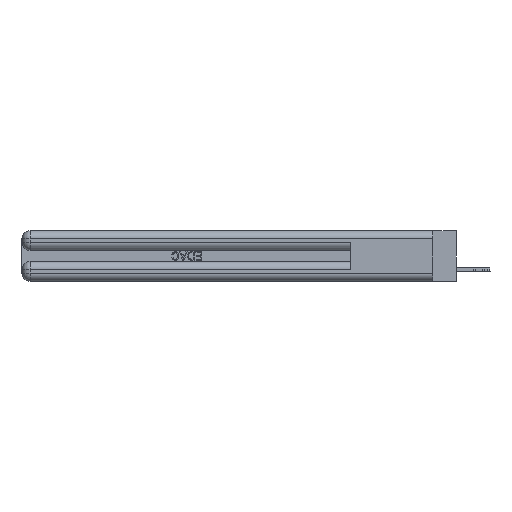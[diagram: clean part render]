
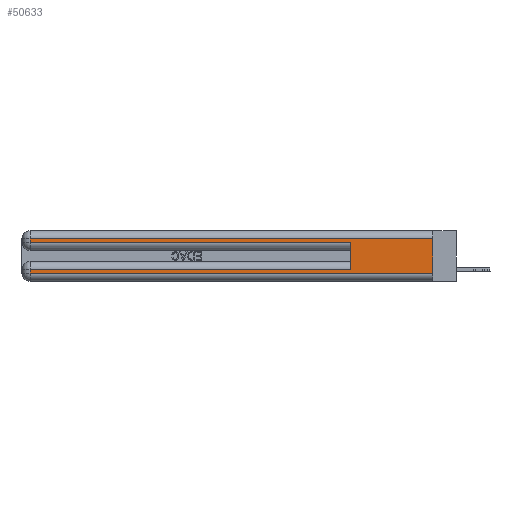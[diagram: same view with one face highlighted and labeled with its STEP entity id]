
A CAD part, left-side view. The second image highlights one B-rep face of the part: STEP entity #50633.
In plain terms, the highlighted planar face has unit normal (-1, 0, 0).
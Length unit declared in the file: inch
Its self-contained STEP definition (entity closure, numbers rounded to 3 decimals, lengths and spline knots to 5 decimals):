
#714 = VERTEX_POINT ( 'NONE', #5975 ) ;
#1698 = DIRECTION ( 'NONE',  ( 0., 0., -1. ) ) ;
#1939 = PLANE ( 'NONE',  #7676 ) ;
#3007 = EDGE_CURVE ( 'NONE', #8865, #45601, #22448, .T. ) ;
#3083 = CARTESIAN_POINT ( 'NONE',  ( 0., 0., 0.37 ) ) ;
#3136 = VECTOR ( 'NONE', #39559, 39.37008 ) ;
#4416 = LINE ( 'NONE', #47238, #3136 ) ;
#5319 = LINE ( 'NONE', #34522, #34477 ) ;
#5425 = VERTEX_POINT ( 'NONE', #7250 ) ;
#5836 = CARTESIAN_POINT ( 'NONE',  ( 0., 2.94, 0.37 ) ) ;
#5975 = CARTESIAN_POINT ( 'NONE',  ( 0., 2.94, 0.06 ) ) ;
#6812 = CARTESIAN_POINT ( 'NONE',  ( 0., 0., 0.31 ) ) ;
#7250 = CARTESIAN_POINT ( 'NONE',  ( 0., 2.94, 0.31 ) ) ;
#7676 = AXIS2_PLACEMENT_3D ( 'NONE', #3083, #44331, #23561 ) ;
#8230 = DIRECTION ( 'NONE',  ( 0., -1., 0. ) ) ;
#8388 = EDGE_CURVE ( 'NONE', #8865, #5425, #21188, .T. ) ;
#8865 = VERTEX_POINT ( 'NONE', #32283 ) ;
#9488 = DIRECTION ( 'NONE',  ( 0., 0., -1. ) ) ;
#10222 = LINE ( 'NONE', #5836, #36821 ) ;
#10442 = CARTESIAN_POINT ( 'NONE',  ( 0., 0., 0.285 ) ) ;
#12274 = DIRECTION ( 'NONE',  ( 0., 1., 0. ) ) ;
#14746 = LINE ( 'NONE', #10442, #50846 ) ;
#15194 = LINE ( 'NONE', #31770, #40395 ) ;
#18966 = CARTESIAN_POINT ( 'NONE',  ( 0., 0., 0.37 ) ) ;
#20331 = EDGE_LOOP ( 'NONE', ( #33616, #41863, #33061, #52438, #41992, #24091, #39143, #36077 ) ) ;
#20453 = VERTEX_POINT ( 'NONE', #47409 ) ;
#20526 = EDGE_CURVE ( 'NONE', #20453, #39081, #14746, .T. ) ;
#20654 = EDGE_CURVE ( 'NONE', #5425, #20453, #10222, .T. ) ;
#21188 = LINE ( 'NONE', #6812, #49023 ) ;
#22448 = LINE ( 'NONE', #18966, #41895 ) ;
#23075 = EDGE_CURVE ( 'NONE', #43983, #714, #5319, .T. ) ;
#23313 = DIRECTION ( 'NONE',  ( 0., 1., 0. ) ) ;
#23561 = DIRECTION ( 'NONE',  ( 0., 0., -1. ) ) ;
#23565 = CARTESIAN_POINT ( 'NONE',  ( 0., 2.94, 0.085 ) ) ;
#24091 = ORIENTED_EDGE ( 'NONE', *, *, #29529, .T. ) ;
#25973 = EDGE_CURVE ( 'NONE', #32829, #39081, #4416, .T. ) ;
#27393 = LINE ( 'NONE', #28270, #36499 ) ;
#28270 = CARTESIAN_POINT ( 'NONE',  ( 0., 0., 0.085 ) ) ;
#29035 = EDGE_CURVE ( 'NONE', #714, #45601, #15194, .T. ) ;
#29337 = CARTESIAN_POINT ( 'NONE',  ( 0., 0., 0.06 ) ) ;
#29529 = EDGE_CURVE ( 'NONE', #32829, #43983, #27393, .T. ) ;
#31770 = CARTESIAN_POINT ( 'NONE',  ( 0., 0., 0.06 ) ) ;
#32283 = CARTESIAN_POINT ( 'NONE',  ( 0., 0., 0.31 ) ) ;
#32829 = VERTEX_POINT ( 'NONE', #52883 ) ;
#33061 = ORIENTED_EDGE ( 'NONE', *, *, #20654, .T. ) ;
#33616 = ORIENTED_EDGE ( 'NONE', *, *, #3007, .F. ) ;
#34477 = VECTOR ( 'NONE', #1698, 39.37008 ) ;
#34522 = CARTESIAN_POINT ( 'NONE',  ( 0., 2.94, 0.37 ) ) ;
#36077 = ORIENTED_EDGE ( 'NONE', *, *, #29035, .T. ) ;
#36499 = VECTOR ( 'NONE', #23313, 39.37008 ) ;
#36821 = VECTOR ( 'NONE', #9488, 39.37008 ) ;
#36904 = FACE_OUTER_BOUND ( 'NONE', #20331, .T. ) ;
#39081 = VERTEX_POINT ( 'NONE', #50231 ) ;
#39143 = ORIENTED_EDGE ( 'NONE', *, *, #23075, .T. ) ;
#39559 = DIRECTION ( 'NONE',  ( 0., 0., 1. ) ) ;
#40395 = VECTOR ( 'NONE', #8230, 39.37008 ) ;
#41863 = ORIENTED_EDGE ( 'NONE', *, *, #8388, .T. ) ;
#41895 = VECTOR ( 'NONE', #51984, 39.37008 ) ;
#41992 = ORIENTED_EDGE ( 'NONE', *, *, #25973, .F. ) ;
#43460 = DIRECTION ( 'NONE',  ( 0., -1., 0. ) ) ;
#43983 = VERTEX_POINT ( 'NONE', #23565 ) ;
#44331 = DIRECTION ( 'NONE',  ( 1., 0., 0. ) ) ;
#45601 = VERTEX_POINT ( 'NONE', #29337 ) ;
#47238 = CARTESIAN_POINT ( 'NONE',  ( 0., 0.6, 0.145 ) ) ;
#47409 = CARTESIAN_POINT ( 'NONE',  ( 0., 2.94, 0.285 ) ) ;
#49023 = VECTOR ( 'NONE', #12274, 39.37008 ) ;
#50231 = CARTESIAN_POINT ( 'NONE',  ( 0., 0.6, 0.285 ) ) ;
#50633 = ADVANCED_FACE ( 'NONE', ( #36904 ), #1939, .F. ) ;
#50846 = VECTOR ( 'NONE', #43460, 39.37008 ) ;
#51984 = DIRECTION ( 'NONE',  ( 0., 0., -1. ) ) ;
#52438 = ORIENTED_EDGE ( 'NONE', *, *, #20526, .T. ) ;
#52883 = CARTESIAN_POINT ( 'NONE',  ( 0., 0.6, 0.085 ) ) ;
